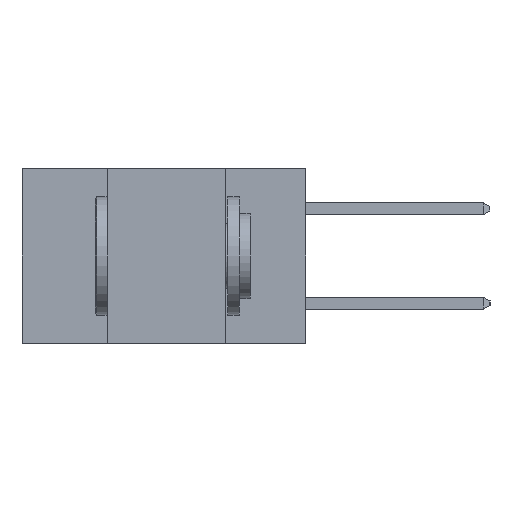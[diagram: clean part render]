
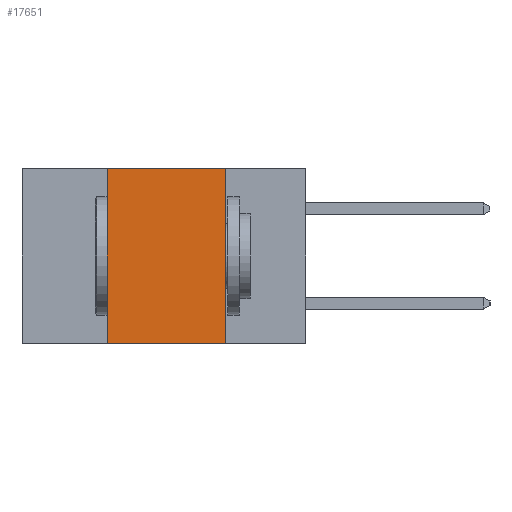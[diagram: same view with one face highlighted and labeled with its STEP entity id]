
A CAD part, left-side view. The second image highlights one B-rep face of the part: STEP entity #17651.
In plain terms, the highlighted planar face has unit normal (-1, 0, 0).
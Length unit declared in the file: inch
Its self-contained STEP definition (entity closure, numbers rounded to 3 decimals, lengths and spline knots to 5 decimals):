
#683 = CARTESIAN_POINT ( 'NONE',  ( 0., 0.42, -0.37 ) ) ;
#727 = VECTOR ( 'NONE', #17809, 39.37008 ) ;
#2941 = ORIENTED_EDGE ( 'NONE', *, *, #11143, .F. ) ;
#3893 = CARTESIAN_POINT ( 'NONE',  ( 0., 0.42, -0.37 ) ) ;
#4181 = CARTESIAN_POINT ( 'NONE',  ( 0., 0.6, -0.37 ) ) ;
#4471 = DIRECTION ( 'NONE',  ( 1., 0., 0. ) ) ;
#4668 = CARTESIAN_POINT ( 'NONE',  ( 0., 0.17, -0.37 ) ) ;
#5483 = CARTESIAN_POINT ( 'NONE',  ( 0., 0.17, -0.37 ) ) ;
#5591 = DIRECTION ( 'NONE',  ( 0., 0., 1. ) ) ;
#6816 = LINE ( 'NONE', #12710, #19302 ) ;
#9943 = LINE ( 'NONE', #4181, #13804 ) ;
#10073 = VERTEX_POINT ( 'NONE', #683 ) ;
#11099 = CARTESIAN_POINT ( 'NONE',  ( 0., 0.6, 0. ) ) ;
#11143 = EDGE_CURVE ( 'NONE', #12315, #13095, #6816, .T. ) ;
#11186 = VECTOR ( 'NONE', #5591, 39.37008 ) ;
#11696 = LINE ( 'NONE', #3893, #11186 ) ;
#12315 = VERTEX_POINT ( 'NONE', #19557 ) ;
#12710 = CARTESIAN_POINT ( 'NONE',  ( 0., 0.6, 0. ) ) ;
#12793 = FACE_OUTER_BOUND ( 'NONE', #15781, .T. ) ;
#13095 = VERTEX_POINT ( 'NONE', #13243 ) ;
#13243 = CARTESIAN_POINT ( 'NONE',  ( 0., 0.17, 0. ) ) ;
#13256 = ORIENTED_EDGE ( 'NONE', *, *, #20212, .F. ) ;
#13782 = DIRECTION ( 'NONE',  ( 0., -1., 0. ) ) ;
#13804 = VECTOR ( 'NONE', #17351, 39.37008 ) ;
#14043 = VERTEX_POINT ( 'NONE', #5483 ) ;
#15781 = EDGE_LOOP ( 'NONE', ( #13256, #2941, #19669, #20424 ) ) ;
#16003 = DIRECTION ( 'NONE',  ( 0., 0., -1. ) ) ;
#17351 = DIRECTION ( 'NONE',  ( 0., -1., 0. ) ) ;
#17528 = EDGE_CURVE ( 'NONE', #10073, #14043, #9943, .T. ) ;
#17542 = PLANE ( 'NONE',  #21048 ) ;
#17651 = ADVANCED_FACE ( 'NONE', ( #12793 ), #17542, .F. ) ;
#17809 = DIRECTION ( 'NONE',  ( 0., 0., -1. ) ) ;
#18253 = LINE ( 'NONE', #4668, #727 ) ;
#19261 = EDGE_CURVE ( 'NONE', #10073, #12315, #11696, .T. ) ;
#19302 = VECTOR ( 'NONE', #13782, 39.37008 ) ;
#19557 = CARTESIAN_POINT ( 'NONE',  ( 0., 0.42, 0. ) ) ;
#19669 = ORIENTED_EDGE ( 'NONE', *, *, #19261, .F. ) ;
#20212 = EDGE_CURVE ( 'NONE', #13095, #14043, #18253, .T. ) ;
#20424 = ORIENTED_EDGE ( 'NONE', *, *, #17528, .T. ) ;
#21048 = AXIS2_PLACEMENT_3D ( 'NONE', #11099, #4471, #16003 ) ;
